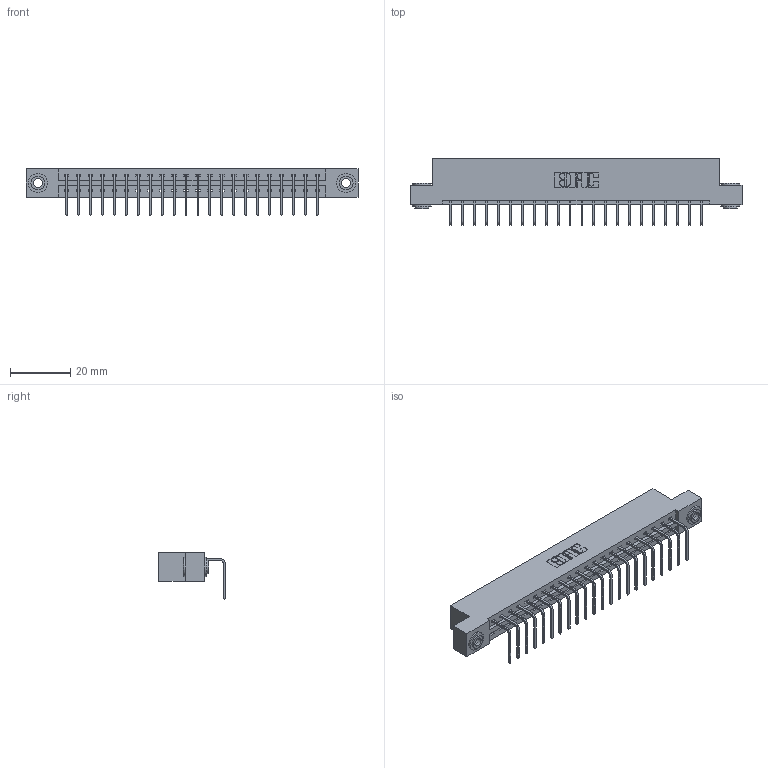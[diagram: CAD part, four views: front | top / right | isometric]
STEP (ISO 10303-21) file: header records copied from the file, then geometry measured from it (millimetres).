
FILE_DESCRIPTION (( 'STEP AP203' ), '1' );
FILE_NAME ('337-022-558-103.STEP', '2019-10-07T12:41:06', ( '' ), ( '' ), 'SwSTEP 2.0', 'SolidWorks 2016', '' );
FILE_SCHEMA (( 'CONFIG_CONTROL_DESIGN' ));
Length unit declared in the file: inch
Products named in the file (4): 337-022-558-103; 345-292-001_558 Tail - 2; 337 Part_Flush Mounting Lugs - 0.156 Dia-TH; 345-250-002_345-250-002-102
Assembly tree (25 placements, depth 2):
  337-022-558-103
    337 Part_Flush Mounting Lugs - 0.156 Dia-TH
    345-292-001_558 Tail - 2  x22
    345-250-002_345-250-002-102  x2
Bounding box: 110.19 x 22.17 x 15.37 mm (x, y, z)
Volume: 11294.3 mm3; surface area: 12243 mm2
Topology: 25 solids, 25 shells, 1560 faces, 4655 edges, 3070 vertices
Faces by surface type: plane 1136, cylinder 416, cone 8
Entity records: 19674 total; most frequent: CARTESIAN_POINT 3403, ORIENTED_EDGE 3354, DIRECTION 2939, EDGE_CURVE 1677, LINE 1525, VECTOR 1525, VERTEX_POINT 1114, AXIS2_PLACEMENT_3D 707
